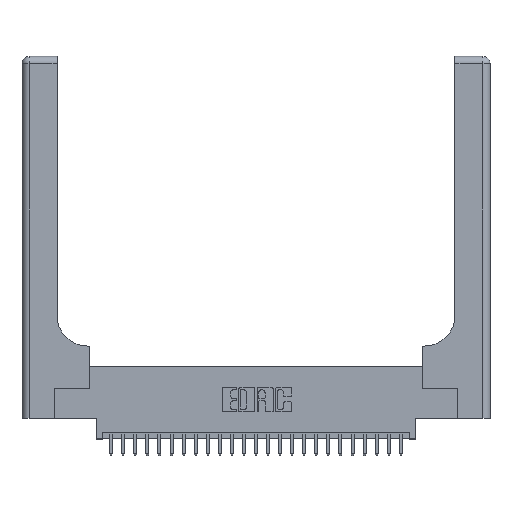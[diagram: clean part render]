
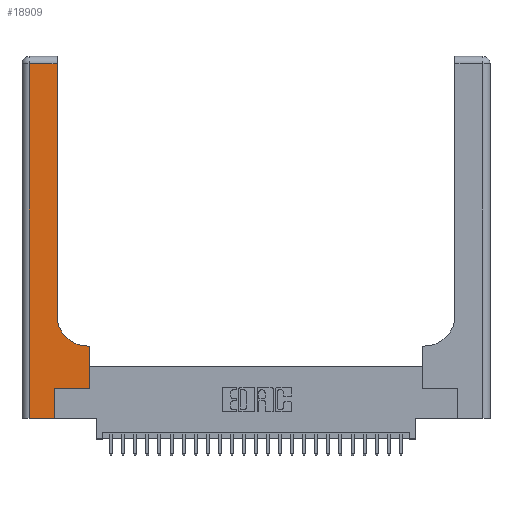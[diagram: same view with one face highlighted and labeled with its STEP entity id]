
A CAD part, top view. The second image highlights one B-rep face of the part: STEP entity #18909.
In plain terms, the highlighted planar face has unit normal (0, 0, 1).
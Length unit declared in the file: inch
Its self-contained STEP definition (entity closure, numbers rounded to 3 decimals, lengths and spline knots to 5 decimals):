
#302 = ORIENTED_EDGE ( 'NONE', *, *, #11264, .T. ) ;
#564 = CARTESIAN_POINT ( 'NONE',  ( 0.5585, 0.25, 0.37 ) ) ;
#1691 = EDGE_CURVE ( 'NONE', #11106, #7254, #19099, .T. ) ;
#1873 = CARTESIAN_POINT ( 'NONE',  ( 0.5585, 0.25, 0.37 ) ) ;
#1991 = VECTOR ( 'NONE', #17403, 39.37008 ) ;
#2274 = VERTEX_POINT ( 'NONE', #22346 ) ;
#2335 = LINE ( 'NONE', #23741, #1991 ) ;
#3077 = VECTOR ( 'NONE', #10627, 39.37008 ) ;
#4123 = CARTESIAN_POINT ( 'NONE',  ( 0.06, 0., 0.37 ) ) ;
#5608 = EDGE_CURVE ( 'NONE', #2274, #6649, #22529, .T. ) ;
#5653 = VERTEX_POINT ( 'NONE', #13616 ) ;
#5720 = DIRECTION ( 'NONE',  ( 0., 0., -1. ) ) ;
#5908 = ORIENTED_EDGE ( 'NONE', *, *, #19481, .T. ) ;
#6037 = VECTOR ( 'NONE', #12830, 39.37008 ) ;
#6175 = CARTESIAN_POINT ( 'NONE',  ( 0.2915, 3., 0.37 ) ) ;
#6644 = CARTESIAN_POINT ( 'NONE',  ( 0.2915, 0.85, 0.37 ) ) ;
#6649 = VERTEX_POINT ( 'NONE', #6644 ) ;
#7254 = VERTEX_POINT ( 'NONE', #4123 ) ;
#8550 = CARTESIAN_POINT ( 'NONE',  ( 0.06, 3., 0.37 ) ) ;
#8894 = EDGE_LOOP ( 'NONE', ( #9035, #22167, #22240, #15326, #5908, #302, #19435, #26135, #13314 ) ) ;
#9035 = ORIENTED_EDGE ( 'NONE', *, *, #24725, .T. ) ;
#9128 = VECTOR ( 'NONE', #20708, 39.37008 ) ;
#10627 = DIRECTION ( 'NONE',  ( 0., 1., 0. ) ) ;
#10867 = CARTESIAN_POINT ( 'NONE',  ( 0.269, 0., 0.37 ) ) ;
#11034 = CARTESIAN_POINT ( 'NONE',  ( 0.269, 0., 0.37 ) ) ;
#11106 = VERTEX_POINT ( 'NONE', #26589 ) ;
#11264 = EDGE_CURVE ( 'NONE', #22844, #26318, #13576, .T. ) ;
#11402 = DIRECTION ( 'NONE',  ( 1., 0., 0. ) ) ;
#11708 = PLANE ( 'NONE',  #22193 ) ;
#12830 = DIRECTION ( 'NONE',  ( -1., 0., 0. ) ) ;
#12963 = DIRECTION ( 'NONE',  ( 0., -1., 0. ) ) ;
#13314 = ORIENTED_EDGE ( 'NONE', *, *, #5608, .T. ) ;
#13576 = LINE ( 'NONE', #18573, #17828 ) ;
#13616 = CARTESIAN_POINT ( 'NONE',  ( 0.5585, 0.6, 0.37 ) ) ;
#13777 = VECTOR ( 'NONE', #17461, 39.37008 ) ;
#13827 = CARTESIAN_POINT ( 'NONE',  ( 0., 3., 0.37 ) ) ;
#13918 = VECTOR ( 'NONE', #18366, 39.37008 ) ;
#14196 = VECTOR ( 'NONE', #12963, 39.37008 ) ;
#14205 = VERTEX_POINT ( 'NONE', #10867 ) ;
#15326 = ORIENTED_EDGE ( 'NONE', *, *, #21088, .T. ) ;
#16075 = CARTESIAN_POINT ( 'NONE',  ( 0., 0., 0.37 ) ) ;
#16894 = EDGE_CURVE ( 'NONE', #5653, #2274, #2335, .T. ) ;
#17403 = DIRECTION ( 'NONE',  ( -1., 0., 0. ) ) ;
#17461 = DIRECTION ( 'NONE',  ( 0., 1., 0. ) ) ;
#17828 = VECTOR ( 'NONE', #24729, 39.37008 ) ;
#17878 = LINE ( 'NONE', #1873, #3077 ) ;
#18319 = LINE ( 'NONE', #6175, #9128 ) ;
#18366 = DIRECTION ( 'NONE',  ( 1., 0., 0. ) ) ;
#18493 = LINE ( 'NONE', #16075, #13918 ) ;
#18543 = CARTESIAN_POINT ( 'NONE',  ( 0.269, 0.25, 0.37 ) ) ;
#18573 = CARTESIAN_POINT ( 'NONE',  ( 0.269, 0.25, 0.37 ) ) ;
#18909 = ADVANCED_FACE ( 'NONE', ( #23613 ), #11708, .F. ) ;
#19099 = LINE ( 'NONE', #8550, #14196 ) ;
#19435 = ORIENTED_EDGE ( 'NONE', *, *, #20337, .T. ) ;
#19481 = EDGE_CURVE ( 'NONE', #14205, #22844, #19680, .T. ) ;
#19680 = LINE ( 'NONE', #11034, #13777 ) ;
#20043 = CARTESIAN_POINT ( 'NONE',  ( 0.5415, 0.85, 0.37 ) ) ;
#20337 = EDGE_CURVE ( 'NONE', #26318, #5653, #17878, .T. ) ;
#20404 = EDGE_CURVE ( 'NONE', #20648, #11106, #25759, .T. ) ;
#20648 = VERTEX_POINT ( 'NONE', #22462 ) ;
#20708 = DIRECTION ( 'NONE',  ( 0., 1., 0. ) ) ;
#21088 = EDGE_CURVE ( 'NONE', #7254, #14205, #18493, .T. ) ;
#22141 = DIRECTION ( 'NONE',  ( 0., 0., -1. ) ) ;
#22167 = ORIENTED_EDGE ( 'NONE', *, *, #20404, .T. ) ;
#22193 = AXIS2_PLACEMENT_3D ( 'NONE', #13827, #5720, #22547 ) ;
#22240 = ORIENTED_EDGE ( 'NONE', *, *, #1691, .T. ) ;
#22346 = CARTESIAN_POINT ( 'NONE',  ( 0.5415, 0.6, 0.37 ) ) ;
#22462 = CARTESIAN_POINT ( 'NONE',  ( 0.2915, 2.94, 0.37 ) ) ;
#22529 = CIRCLE ( 'NONE', #25021, 0.25 ) ;
#22547 = DIRECTION ( 'NONE',  ( -1., 0., 0. ) ) ;
#22844 = VERTEX_POINT ( 'NONE', #18543 ) ;
#23613 = FACE_OUTER_BOUND ( 'NONE', #8894, .T. ) ;
#23741 = CARTESIAN_POINT ( 'NONE',  ( 0.2915, 0.6, 0.37 ) ) ;
#24725 = EDGE_CURVE ( 'NONE', #6649, #20648, #18319, .T. ) ;
#24729 = DIRECTION ( 'NONE',  ( 1., 0., 0. ) ) ;
#25021 = AXIS2_PLACEMENT_3D ( 'NONE', #20043, #22141, #11402 ) ;
#25416 = CARTESIAN_POINT ( 'NONE',  ( 0., 2.94, 0.37 ) ) ;
#25759 = LINE ( 'NONE', #25416, #6037 ) ;
#26135 = ORIENTED_EDGE ( 'NONE', *, *, #16894, .T. ) ;
#26318 = VERTEX_POINT ( 'NONE', #564 ) ;
#26589 = CARTESIAN_POINT ( 'NONE',  ( 0.06, 2.94, 0.37 ) ) ;
